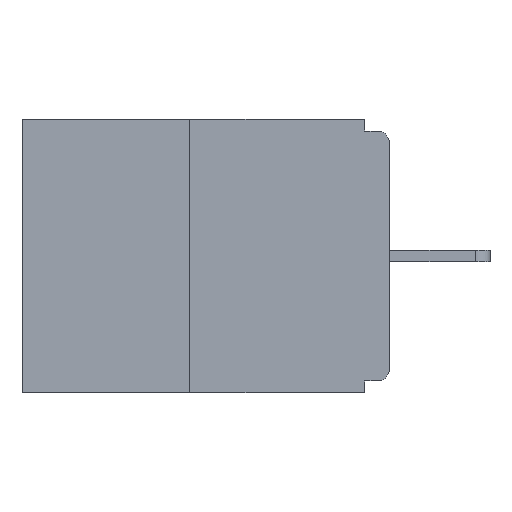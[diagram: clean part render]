
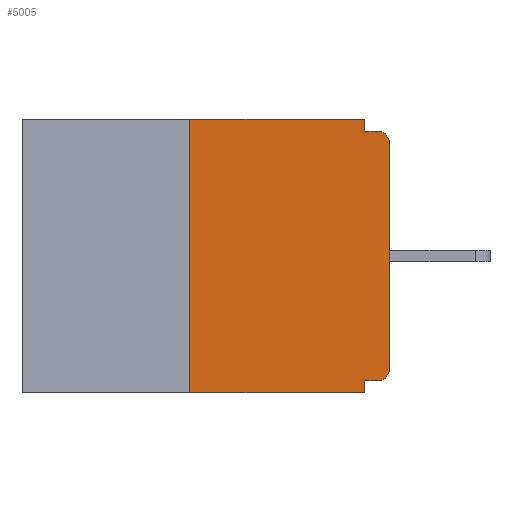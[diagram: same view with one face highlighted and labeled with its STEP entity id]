
A CAD part, left-side view. The second image highlights one B-rep face of the part: STEP entity #5005.
In plain terms, the highlighted planar face has unit normal (-1, 0, 0).
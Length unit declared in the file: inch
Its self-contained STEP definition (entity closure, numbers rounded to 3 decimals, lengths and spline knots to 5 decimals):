
#82 = VERTEX_POINT ( 'NONE', #13235 ) ;
#229 = DIRECTION ( 'NONE',  ( 1., 0., 0. ) ) ;
#415 = CARTESIAN_POINT ( 'NONE',  ( 0., 0.015, -0.328 ) ) ;
#642 = VERTEX_POINT ( 'NONE', #15175 ) ;
#863 = VERTEX_POINT ( 'NONE', #1487 ) ;
#1268 = VERTEX_POINT ( 'NONE', #7809 ) ;
#1325 = EDGE_CURVE ( 'NONE', #1415, #642, #10363, .T. ) ;
#1415 = VERTEX_POINT ( 'NONE', #3241 ) ;
#1471 = CARTESIAN_POINT ( 'NONE',  ( 0., 0.46, 0. ) ) ;
#1487 = CARTESIAN_POINT ( 'NONE',  ( 0., 0.031, -0.328 ) ) ;
#1631 = CARTESIAN_POINT ( 'NONE',  ( 0., 0.46, -0.343 ) ) ;
#2290 = VECTOR ( 'NONE', #4411, 39.37008 ) ;
#2673 = EDGE_CURVE ( 'NONE', #13853, #642, #7448, .T. ) ;
#2823 = ORIENTED_EDGE ( 'NONE', *, *, #14113, .T. ) ;
#3231 = LINE ( 'NONE', #4850, #14557 ) ;
#3241 = CARTESIAN_POINT ( 'NONE',  ( 0., 0.031, -0.015 ) ) ;
#3270 = VERTEX_POINT ( 'NONE', #18083 ) ;
#3299 = ORIENTED_EDGE ( 'NONE', *, *, #14030, .F. ) ;
#3494 = ORIENTED_EDGE ( 'NONE', *, *, #14670, .F. ) ;
#3921 = CARTESIAN_POINT ( 'NONE',  ( 0., 0.46, 0. ) ) ;
#4001 = VECTOR ( 'NONE', #14509, 39.37008 ) ;
#4153 = EDGE_CURVE ( 'NONE', #1268, #1415, #14629, .T. ) ;
#4192 = FACE_OUTER_BOUND ( 'NONE', #7390, .T. ) ;
#4411 = DIRECTION ( 'NONE',  ( 0., -1., 0. ) ) ;
#4454 = LINE ( 'NONE', #1631, #4001 ) ;
#4677 = PLANE ( 'NONE',  #15901 ) ;
#4678 = CARTESIAN_POINT ( 'NONE',  ( 0., 0., -0.015 ) ) ;
#4728 = ORIENTED_EDGE ( 'NONE', *, *, #13443, .F. ) ;
#4850 = CARTESIAN_POINT ( 'NONE',  ( 0., 0.031, -0.343 ) ) ;
#4856 = DIRECTION ( 'NONE',  ( -1., 0., 0. ) ) ;
#5005 = ADVANCED_FACE ( 'NONE', ( #4192 ), #4677, .F. ) ;
#5239 = VERTEX_POINT ( 'NONE', #7766 ) ;
#5289 = LINE ( 'NONE', #9099, #12366 ) ;
#5364 = CIRCLE ( 'NONE', #12199, 0.015 ) ;
#6129 = ORIENTED_EDGE ( 'NONE', *, *, #14132, .T. ) ;
#6759 = DIRECTION ( 'NONE',  ( 0., 0., -1. ) ) ;
#6789 = CARTESIAN_POINT ( 'NONE',  ( 0., 0., -0.03 ) ) ;
#6835 = DIRECTION ( 'NONE',  ( -1., 0., 0. ) ) ;
#6967 = CARTESIAN_POINT ( 'NONE',  ( 0., 0.015, -0.03 ) ) ;
#7052 = ORIENTED_EDGE ( 'NONE', *, *, #2673, .T. ) ;
#7305 = CARTESIAN_POINT ( 'NONE',  ( 0., 0.25, 0. ) ) ;
#7390 = EDGE_LOOP ( 'NONE', ( #3494, #4728, #6129, #17039, #3299, #2823, #10802, #7052, #12128, #15202 ) ) ;
#7448 = CIRCLE ( 'NONE', #16777, 0.015 ) ;
#7497 = CARTESIAN_POINT ( 'NONE',  ( 0., 0.25, 0. ) ) ;
#7766 = CARTESIAN_POINT ( 'NONE',  ( 0., 0.25, -0.343 ) ) ;
#7809 = CARTESIAN_POINT ( 'NONE',  ( 0., 0.031, 0. ) ) ;
#8727 = DIRECTION ( 'NONE',  ( 0., -1., 0. ) ) ;
#9099 = CARTESIAN_POINT ( 'NONE',  ( 0., 0., 0. ) ) ;
#9149 = VECTOR ( 'NONE', #15645, 39.37008 ) ;
#9341 = LINE ( 'NONE', #1471, #12635 ) ;
#9493 = EDGE_CURVE ( 'NONE', #3270, #13853, #5289, .T. ) ;
#10267 = DIRECTION ( 'NONE',  ( 0., 0., -1. ) ) ;
#10363 = LINE ( 'NONE', #4678, #2290 ) ;
#10512 = DIRECTION ( 'NONE',  ( 0., 0., 1. ) ) ;
#10802 = ORIENTED_EDGE ( 'NONE', *, *, #9493, .T. ) ;
#11629 = CARTESIAN_POINT ( 'NONE',  ( 0., 0.015, -0.313 ) ) ;
#11939 = CARTESIAN_POINT ( 'NONE',  ( 0., 0.031, 0. ) ) ;
#11961 = DIRECTION ( 'NONE',  ( 0., 0., -1. ) ) ;
#12128 = ORIENTED_EDGE ( 'NONE', *, *, #1325, .F. ) ;
#12199 = AXIS2_PLACEMENT_3D ( 'NONE', #11629, #4856, #10267 ) ;
#12366 = VECTOR ( 'NONE', #10512, 39.37008 ) ;
#12464 = VERTEX_POINT ( 'NONE', #415 ) ;
#12635 = VECTOR ( 'NONE', #8727, 39.37008 ) ;
#12874 = CARTESIAN_POINT ( 'NONE',  ( 0., 0., -0.328 ) ) ;
#12886 = LINE ( 'NONE', #12874, #9149 ) ;
#13235 = CARTESIAN_POINT ( 'NONE',  ( 0., 0.031, -0.343 ) ) ;
#13339 = DIRECTION ( 'NONE',  ( 0., 0., -1. ) ) ;
#13443 = EDGE_CURVE ( 'NONE', #5239, #18107, #15500, .T. ) ;
#13853 = VERTEX_POINT ( 'NONE', #6789 ) ;
#14030 = EDGE_CURVE ( 'NONE', #12464, #863, #12886, .T. ) ;
#14113 = EDGE_CURVE ( 'NONE', #12464, #3270, #5364, .T. ) ;
#14132 = EDGE_CURVE ( 'NONE', #5239, #82, #4454, .T. ) ;
#14509 = DIRECTION ( 'NONE',  ( 0., -1., 0. ) ) ;
#14557 = VECTOR ( 'NONE', #13339, 39.37008 ) ;
#14629 = LINE ( 'NONE', #11939, #15055 ) ;
#14670 = EDGE_CURVE ( 'NONE', #18107, #1268, #9341, .T. ) ;
#15055 = VECTOR ( 'NONE', #11961, 39.37008 ) ;
#15175 = CARTESIAN_POINT ( 'NONE',  ( 0., 0.015, -0.015 ) ) ;
#15202 = ORIENTED_EDGE ( 'NONE', *, *, #4153, .F. ) ;
#15500 = LINE ( 'NONE', #7305, #15918 ) ;
#15577 = DIRECTION ( 'NONE',  ( 0., 0., -1. ) ) ;
#15645 = DIRECTION ( 'NONE',  ( 0., 1., 0. ) ) ;
#15901 = AXIS2_PLACEMENT_3D ( 'NONE', #3921, #229, #15577 ) ;
#15918 = VECTOR ( 'NONE', #17017, 39.37008 ) ;
#16056 = EDGE_CURVE ( 'NONE', #863, #82, #3231, .T. ) ;
#16777 = AXIS2_PLACEMENT_3D ( 'NONE', #6967, #6835, #6759 ) ;
#17017 = DIRECTION ( 'NONE',  ( 0., 0., 1. ) ) ;
#17039 = ORIENTED_EDGE ( 'NONE', *, *, #16056, .F. ) ;
#18083 = CARTESIAN_POINT ( 'NONE',  ( 0., 0., -0.313 ) ) ;
#18107 = VERTEX_POINT ( 'NONE', #7497 ) ;
